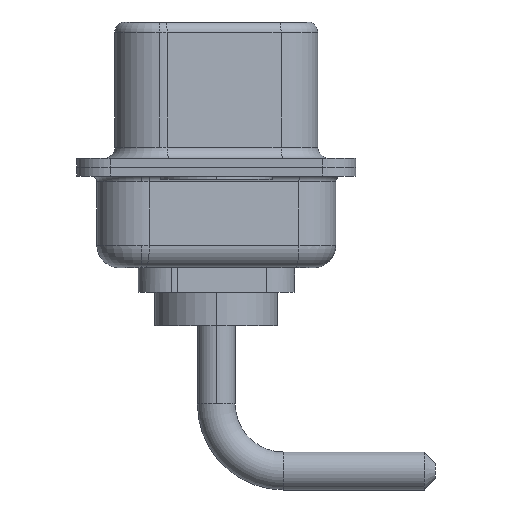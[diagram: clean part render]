
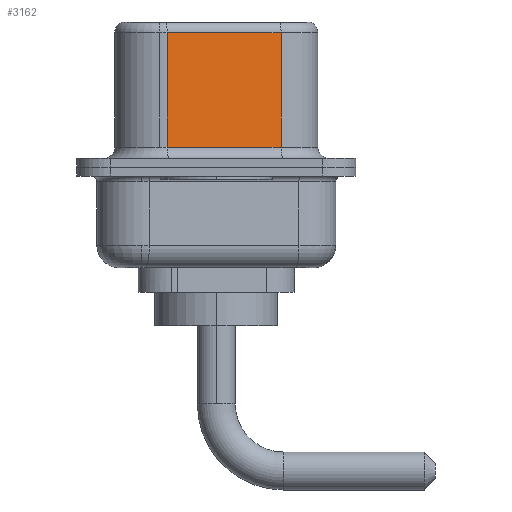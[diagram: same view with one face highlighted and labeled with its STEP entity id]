
A CAD part, left-side view. The second image highlights one B-rep face of the part: STEP entity #3162.
In plain terms, the highlighted planar face has unit normal (-0.985, -0.174, 0).
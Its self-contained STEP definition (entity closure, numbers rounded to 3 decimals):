
#147 = CARTESIAN_POINT ( 'NONE',  ( 4.555, -2.897, 0.9 ) ) ;
#267 = VERTEX_POINT ( 'NONE', #1806 ) ;
#1128 = CARTESIAN_POINT ( 'NONE',  ( 3.655, 2.203, 6.02 ) ) ;
#1251 = CARTESIAN_POINT ( 'NONE',  ( 4.555, -2.897, 6.02 ) ) ;
#1665 = CARTESIAN_POINT ( 'NONE',  ( 3.655, 2.203, 0.9 ) ) ;
#1699 = VECTOR ( 'NONE', #6788, 1000. ) ;
#1806 = CARTESIAN_POINT ( 'NONE',  ( 4.555, -2.897, 0.9 ) ) ;
#2469 = ORIENTED_EDGE ( 'NONE', *, *, #5492, .F. ) ;
#2770 = CARTESIAN_POINT ( 'NONE',  ( 3.655, 2.203, 6.52 ) ) ;
#3108 = AXIS2_PLACEMENT_3D ( 'NONE', #3939, #11583, #9495 ) ;
#3162 = ADVANCED_FACE ( 'NONE', ( #4992 ), #13562, .F. ) ;
#3456 = VERTEX_POINT ( 'NONE', #1665 ) ;
#3841 = VECTOR ( 'NONE', #10372, 1000. ) ;
#3939 = CARTESIAN_POINT ( 'NONE',  ( 4.555, -2.897, 6.52 ) ) ;
#3954 = EDGE_CURVE ( 'NONE', #7632, #3456, #10437, .T. ) ;
#4992 = FACE_OUTER_BOUND ( 'NONE', #11977, .T. ) ;
#5414 = DIRECTION ( 'NONE',  ( 0.174, -0.985, 0. ) ) ;
#5492 = EDGE_CURVE ( 'NONE', #9248, #267, #5581, .T. ) ;
#5581 = LINE ( 'NONE', #12753, #1699 ) ;
#6788 = DIRECTION ( 'NONE',  ( 0., 0., -1. ) ) ;
#6955 = LINE ( 'NONE', #12414, #13395 ) ;
#7163 = ORIENTED_EDGE ( 'NONE', *, *, #9853, .T. ) ;
#7632 = VERTEX_POINT ( 'NONE', #1128 ) ;
#9134 = DIRECTION ( 'NONE',  ( -0.174, 0.985, 0. ) ) ;
#9248 = VERTEX_POINT ( 'NONE', #1251 ) ;
#9280 = EDGE_CURVE ( 'NONE', #3456, #267, #12996, .T. ) ;
#9495 = DIRECTION ( 'NONE',  ( -0.174, 0.985, 0. ) ) ;
#9853 = EDGE_CURVE ( 'NONE', #9248, #7632, #6955, .T. ) ;
#9940 = ORIENTED_EDGE ( 'NONE', *, *, #9280, .T. ) ;
#10372 = DIRECTION ( 'NONE',  ( 0., 0., -1. ) ) ;
#10437 = LINE ( 'NONE', #2770, #3841 ) ;
#11566 = VECTOR ( 'NONE', #5414, 1000. ) ;
#11583 = DIRECTION ( 'NONE',  ( 0.985, 0.174, 0. ) ) ;
#11977 = EDGE_LOOP ( 'NONE', ( #2469, #7163, #13679, #9940 ) ) ;
#12414 = CARTESIAN_POINT ( 'NONE',  ( 4.555, -2.897, 6.02 ) ) ;
#12753 = CARTESIAN_POINT ( 'NONE',  ( 4.555, -2.897, 6.52 ) ) ;
#12996 = LINE ( 'NONE', #147, #11566 ) ;
#13395 = VECTOR ( 'NONE', #9134, 1000. ) ;
#13562 = PLANE ( 'NONE',  #3108 ) ;
#13679 = ORIENTED_EDGE ( 'NONE', *, *, #3954, .T. ) ;
